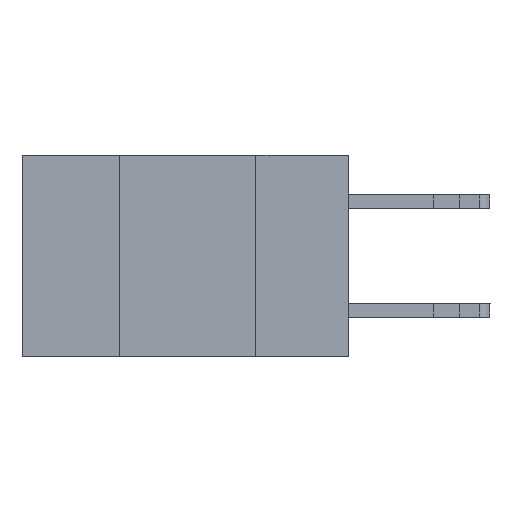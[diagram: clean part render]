
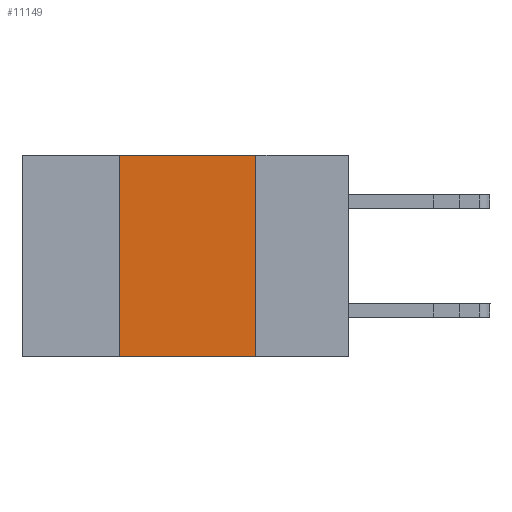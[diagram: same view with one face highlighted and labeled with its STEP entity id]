
A CAD part, left-side view. The second image highlights one B-rep face of the part: STEP entity #11149.
In plain terms, the highlighted planar face has unit normal (-1, 0, 0).
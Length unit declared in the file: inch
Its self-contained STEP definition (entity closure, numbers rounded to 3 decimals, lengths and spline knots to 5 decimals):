
#392 = VERTEX_POINT ( 'NONE', #8913 ) ;
#1275 = LINE ( 'NONE', #6590, #9144 ) ;
#2241 = CARTESIAN_POINT ( 'NONE',  ( 0., 0.17, -0.37 ) ) ;
#2722 = CARTESIAN_POINT ( 'NONE',  ( 0., 0.6, 0. ) ) ;
#2887 = EDGE_LOOP ( 'NONE', ( #15323, #21074, #16311, #17093 ) ) ;
#3109 = EDGE_CURVE ( 'NONE', #25920, #18451, #21751, .T. ) ;
#3113 = CARTESIAN_POINT ( 'NONE',  ( 0., 0.42, 0. ) ) ;
#4904 = DIRECTION ( 'NONE',  ( 0., 0., -1. ) ) ;
#5792 = FACE_OUTER_BOUND ( 'NONE', #2887, .T. ) ;
#6017 = LINE ( 'NONE', #11624, #21730 ) ;
#6122 = VECTOR ( 'NONE', #17834, 39.37008 ) ;
#6590 = CARTESIAN_POINT ( 'NONE',  ( 0., 0.17, 0. ) ) ;
#7844 = DIRECTION ( 'NONE',  ( 0., -1., 0. ) ) ;
#8682 = CARTESIAN_POINT ( 'NONE',  ( 0., 0.42, -0.37 ) ) ;
#8776 = DIRECTION ( 'NONE',  ( 1., 0., 0. ) ) ;
#8913 = CARTESIAN_POINT ( 'NONE',  ( 0., 0.17, 0. ) ) ;
#9144 = VECTOR ( 'NONE', #20661, 39.37008 ) ;
#9671 = AXIS2_PLACEMENT_3D ( 'NONE', #2722, #8776, #4904 ) ;
#11149 = ADVANCED_FACE ( 'NONE', ( #5792 ), #20868, .F. ) ;
#11183 = DIRECTION ( 'NONE',  ( 0., 0., 1. ) ) ;
#11624 = CARTESIAN_POINT ( 'NONE',  ( 0., 0.6, 0. ) ) ;
#11836 = VERTEX_POINT ( 'NONE', #2241 ) ;
#12360 = CARTESIAN_POINT ( 'NONE',  ( 0., 0.42, 0. ) ) ;
#12726 = LINE ( 'NONE', #23808, #6122 ) ;
#15323 = ORIENTED_EDGE ( 'NONE', *, *, #20121, .F. ) ;
#16311 = ORIENTED_EDGE ( 'NONE', *, *, #3109, .F. ) ;
#17093 = ORIENTED_EDGE ( 'NONE', *, *, #24865, .T. ) ;
#17834 = DIRECTION ( 'NONE',  ( 0., -1., 0. ) ) ;
#18451 = VERTEX_POINT ( 'NONE', #12360 ) ;
#18955 = VECTOR ( 'NONE', #11183, 39.37008 ) ;
#20121 = EDGE_CURVE ( 'NONE', #392, #11836, #1275, .T. ) ;
#20392 = EDGE_CURVE ( 'NONE', #18451, #392, #6017, .T. ) ;
#20661 = DIRECTION ( 'NONE',  ( 0., 0., -1. ) ) ;
#20868 = PLANE ( 'NONE',  #9671 ) ;
#21074 = ORIENTED_EDGE ( 'NONE', *, *, #20392, .F. ) ;
#21730 = VECTOR ( 'NONE', #7844, 39.37008 ) ;
#21751 = LINE ( 'NONE', #3113, #18955 ) ;
#23808 = CARTESIAN_POINT ( 'NONE',  ( 0., 0.6, -0.37 ) ) ;
#24865 = EDGE_CURVE ( 'NONE', #25920, #11836, #12726, .T. ) ;
#25920 = VERTEX_POINT ( 'NONE', #8682 ) ;
